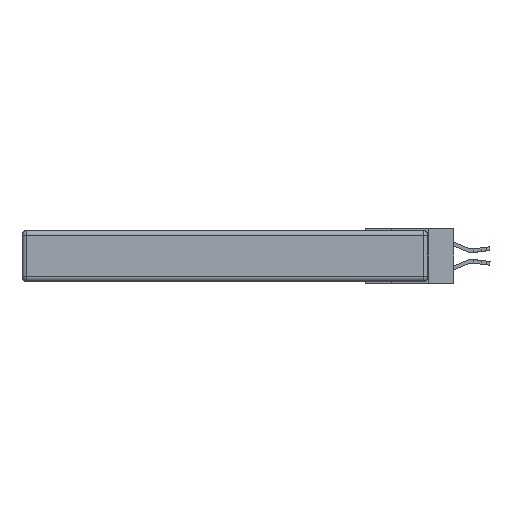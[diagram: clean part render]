
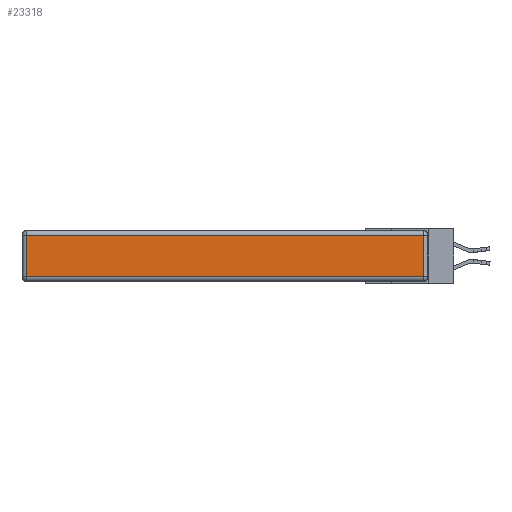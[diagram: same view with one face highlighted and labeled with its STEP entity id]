
A CAD part, left-side view. The second image highlights one B-rep face of the part: STEP entity #23318.
In plain terms, the highlighted planar face has unit normal (-1, 0, 0).
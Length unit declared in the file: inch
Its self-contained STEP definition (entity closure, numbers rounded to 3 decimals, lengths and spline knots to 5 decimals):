
#1591 = EDGE_CURVE ( 'NONE', #6287, #21484, #23944, .T. ) ;
#1962 = ORIENTED_EDGE ( 'NONE', *, *, #1591, .T. ) ;
#3432 = VECTOR ( 'NONE', #4426, 39.37008 ) ;
#4179 = EDGE_CURVE ( 'NONE', #20622, #17848, #4829, .T. ) ;
#4426 = DIRECTION ( 'NONE',  ( 0., -1., 0. ) ) ;
#4829 = LINE ( 'NONE', #13519, #7184 ) ;
#6287 = VERTEX_POINT ( 'NONE', #22626 ) ;
#7184 = VECTOR ( 'NONE', #23984, 39.37008 ) ;
#8257 = ORIENTED_EDGE ( 'NONE', *, *, #13915, .T. ) ;
#9049 = ORIENTED_EDGE ( 'NONE', *, *, #4179, .T. ) ;
#9087 = CARTESIAN_POINT ( 'NONE',  ( 0., 0., -0.343 ) ) ;
#9915 = LINE ( 'NONE', #18255, #10235 ) ;
#10235 = VECTOR ( 'NONE', #18611, 39.37008 ) ;
#10588 = CARTESIAN_POINT ( 'NONE',  ( 0., 0., -0.313 ) ) ;
#11125 = PLANE ( 'NONE',  #22557 ) ;
#11801 = LINE ( 'NONE', #20528, #20052 ) ;
#12058 = DIRECTION ( 'NONE',  ( 0., 0., -1. ) ) ;
#13252 = DIRECTION ( 'NONE',  ( 0., 0., 1. ) ) ;
#13519 = CARTESIAN_POINT ( 'NONE',  ( 0., 2.75, -0.03 ) ) ;
#13849 = CARTESIAN_POINT ( 'NONE',  ( 0., 0.03, -0.313 ) ) ;
#13915 = EDGE_CURVE ( 'NONE', #17848, #6287, #11801, .T. ) ;
#15907 = EDGE_LOOP ( 'NONE', ( #1962, #19791, #9049, #8257 ) ) ;
#17848 = VERTEX_POINT ( 'NONE', #20714 ) ;
#18255 = CARTESIAN_POINT ( 'NONE',  ( 0., 0.03, -0.343 ) ) ;
#18611 = DIRECTION ( 'NONE',  ( 0., 0., 1. ) ) ;
#18954 = CARTESIAN_POINT ( 'NONE',  ( 0., 0.03, -0.03 ) ) ;
#19791 = ORIENTED_EDGE ( 'NONE', *, *, #22860, .T. ) ;
#20052 = VECTOR ( 'NONE', #12058, 39.37008 ) ;
#20528 = CARTESIAN_POINT ( 'NONE',  ( 0., 2.72, -0.343 ) ) ;
#20622 = VERTEX_POINT ( 'NONE', #18954 ) ;
#20714 = CARTESIAN_POINT ( 'NONE',  ( 0., 2.72, -0.03 ) ) ;
#21484 = VERTEX_POINT ( 'NONE', #13849 ) ;
#22557 = AXIS2_PLACEMENT_3D ( 'NONE', #9087, #25862, #13252 ) ;
#22626 = CARTESIAN_POINT ( 'NONE',  ( 0., 2.72, -0.313 ) ) ;
#22860 = EDGE_CURVE ( 'NONE', #21484, #20622, #9915, .T. ) ;
#23318 = ADVANCED_FACE ( 'NONE', ( #23388 ), #11125, .T. ) ;
#23388 = FACE_OUTER_BOUND ( 'NONE', #15907, .T. ) ;
#23944 = LINE ( 'NONE', #10588, #3432 ) ;
#23984 = DIRECTION ( 'NONE',  ( 0., 1., 0. ) ) ;
#25862 = DIRECTION ( 'NONE',  ( -1., 0., 0. ) ) ;
